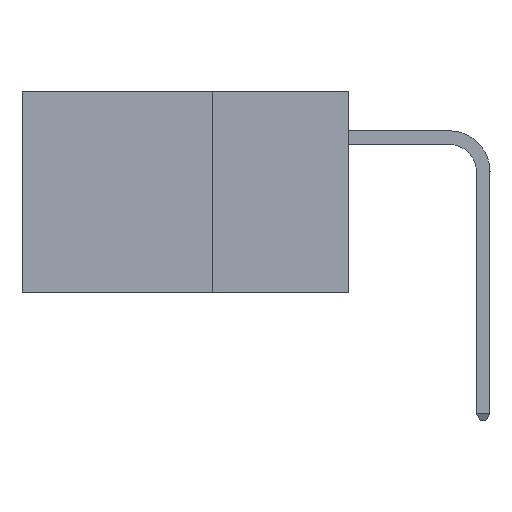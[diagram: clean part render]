
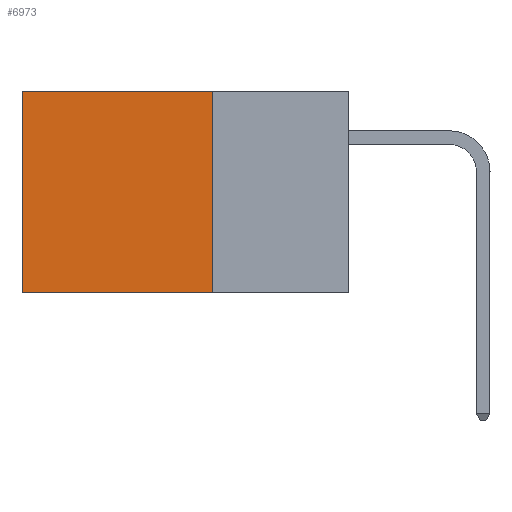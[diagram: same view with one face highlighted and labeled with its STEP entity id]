
A CAD part, left-side view. The second image highlights one B-rep face of the part: STEP entity #6973.
In plain terms, the highlighted planar face has unit normal (-1, 0, 0).
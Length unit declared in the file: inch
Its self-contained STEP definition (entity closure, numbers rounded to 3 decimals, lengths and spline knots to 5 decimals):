
#132 = LINE ( 'NONE', #6342, #8645 ) ;
#191 = CARTESIAN_POINT ( 'NONE',  ( 0.2875, 0.6, 0. ) ) ;
#301 = EDGE_CURVE ( 'NONE', #5927, #7893, #10160, .T. ) ;
#881 = DIRECTION ( 'NONE',  ( 0., 1., 0. ) ) ;
#1015 = ORIENTED_EDGE ( 'NONE', *, *, #5589, .T. ) ;
#1136 = EDGE_CURVE ( 'NONE', #6151, #1959, #6855, .T. ) ;
#1537 = CARTESIAN_POINT ( 'NONE',  ( 0.2875, 0.25, 0. ) ) ;
#1959 = VERTEX_POINT ( 'NONE', #6503 ) ;
#2382 = PLANE ( 'NONE',  #4994 ) ;
#3206 = DIRECTION ( 'NONE',  ( 1., 0., 0. ) ) ;
#4200 = CARTESIAN_POINT ( 'NONE',  ( 0.2875, 0.25, -0.37 ) ) ;
#4331 = ORIENTED_EDGE ( 'NONE', *, *, #301, .T. ) ;
#4489 = EDGE_CURVE ( 'NONE', #1959, #7893, #9693, .T. ) ;
#4858 = ORIENTED_EDGE ( 'NONE', *, *, #1136, .F. ) ;
#4875 = DIRECTION ( 'NONE',  ( 0., 0., -1. ) ) ;
#4890 = CARTESIAN_POINT ( 'NONE',  ( 0.2875, 0.25, 0. ) ) ;
#4994 = AXIS2_PLACEMENT_3D ( 'NONE', #1537, #3206, #8924 ) ;
#5551 = CARTESIAN_POINT ( 'NONE',  ( 0.2875, 0.6, 0. ) ) ;
#5589 = EDGE_CURVE ( 'NONE', #6151, #5927, #132, .T. ) ;
#5597 = DIRECTION ( 'NONE',  ( 0., 0., -1. ) ) ;
#5927 = VERTEX_POINT ( 'NONE', #191 ) ;
#6151 = VERTEX_POINT ( 'NONE', #7860 ) ;
#6173 = CARTESIAN_POINT ( 'NONE',  ( 0.2875, 0.6, -0.37 ) ) ;
#6342 = CARTESIAN_POINT ( 'NONE',  ( 0.2875, 0.25, 0. ) ) ;
#6503 = CARTESIAN_POINT ( 'NONE',  ( 0.2875, 0.25, -0.37 ) ) ;
#6855 = LINE ( 'NONE', #4890, #10621 ) ;
#6973 = ADVANCED_FACE ( 'NONE', ( #10157 ), #2382, .F. ) ;
#7860 = CARTESIAN_POINT ( 'NONE',  ( 0.2875, 0.25, 0. ) ) ;
#7893 = VERTEX_POINT ( 'NONE', #6173 ) ;
#8645 = VECTOR ( 'NONE', #8774, 39.37008 ) ;
#8743 = ORIENTED_EDGE ( 'NONE', *, *, #4489, .F. ) ;
#8774 = DIRECTION ( 'NONE',  ( 0., 1., 0. ) ) ;
#8924 = DIRECTION ( 'NONE',  ( 0., 0., -1. ) ) ;
#9210 = VECTOR ( 'NONE', #881, 39.37008 ) ;
#9247 = EDGE_LOOP ( 'NONE', ( #4331, #8743, #4858, #1015 ) ) ;
#9693 = LINE ( 'NONE', #4200, #9210 ) ;
#9902 = VECTOR ( 'NONE', #5597, 39.37008 ) ;
#10157 = FACE_OUTER_BOUND ( 'NONE', #9247, .T. ) ;
#10160 = LINE ( 'NONE', #5551, #9902 ) ;
#10621 = VECTOR ( 'NONE', #4875, 39.37008 ) ;
